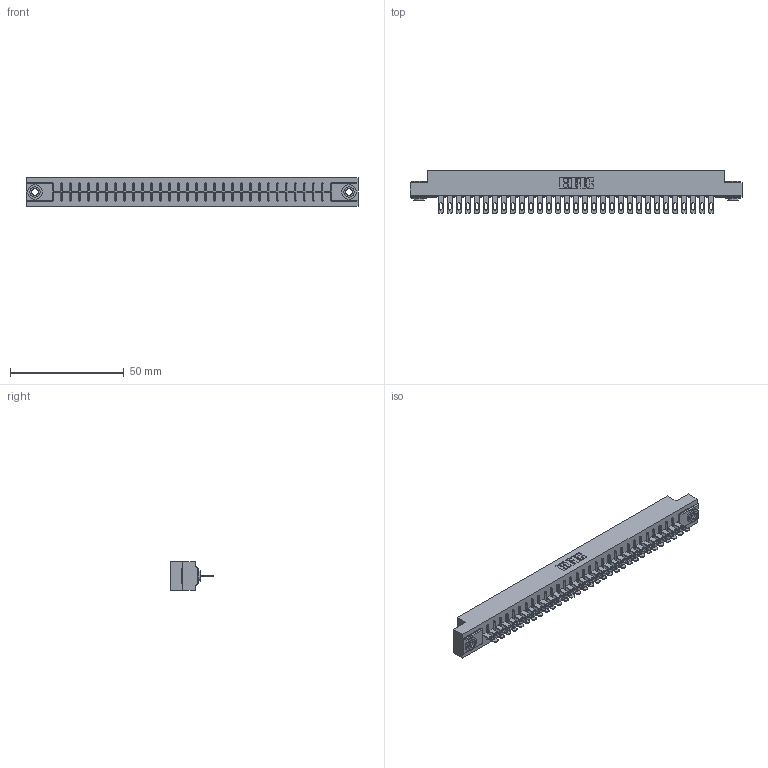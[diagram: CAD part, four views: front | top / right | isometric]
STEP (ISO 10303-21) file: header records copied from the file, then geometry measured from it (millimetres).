
FILE_DESCRIPTION (( 'STEP AP203' ), '1' );
FILE_NAME ('356-031-500-103.STEP', '2018-08-01T21:03:18', ( '' ), ( '' ), 'SwSTEP 2.0', 'SolidWorks 2016', '' );
FILE_SCHEMA (( 'CONFIG_CONTROL_DESIGN' ));
Length unit declared in the file: inch
Products named in the file (4): 306 Part_.156 Dia; 306-290-001_100; 345-250-002_345-250-002-102; 356-031-500-103
Assembly tree (34 placements, depth 2):
  356-031-500-103
    306 Part_.156 Dia
    306-290-001_100  x31
    345-250-002_345-250-002-102  x2
Bounding box: 145.85 x 18.87 x 12.7 mm (x, y, z)
Volume: 16127 mm3; surface area: 17238.8 mm2
Topology: 34 solids, 34 shells, 2524 faces, 7093 edges, 4558 vertices
Faces by surface type: plane 1642, cylinder 750, sphere 124, cone 8
Entity records: 31563 total; most frequent: CARTESIAN_POINT 5277, ORIENTED_EDGE 5222, DIRECTION 5219, EDGE_CURVE 2611, LINE 2027, VECTOR 2027, VERTEX_POINT 1654, AXIS2_PLACEMENT_3D 1596
